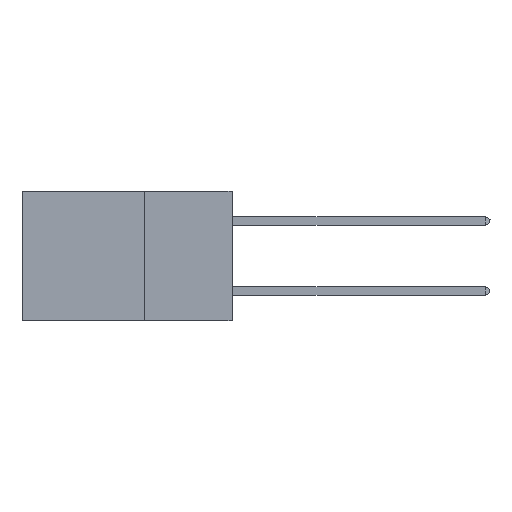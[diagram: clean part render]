
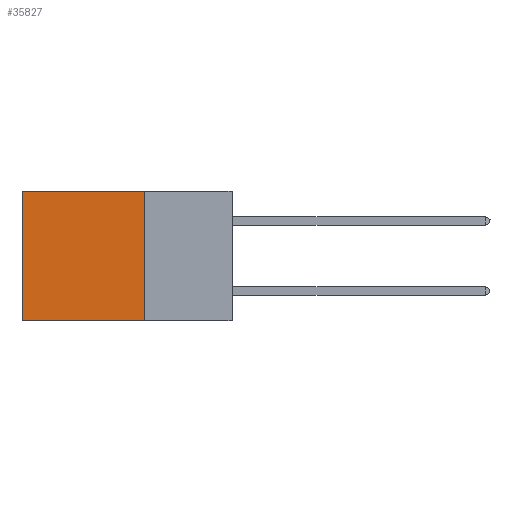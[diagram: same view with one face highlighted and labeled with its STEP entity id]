
A CAD part, left-side view. The second image highlights one B-rep face of the part: STEP entity #35827.
In plain terms, the highlighted planar face has unit normal (-1, 0, 0).
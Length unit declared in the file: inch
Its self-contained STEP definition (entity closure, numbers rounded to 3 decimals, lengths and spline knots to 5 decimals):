
#1956 = LINE ( 'NONE', #14422, #10364 ) ;
#3294 = ORIENTED_EDGE ( 'NONE', *, *, #44660, .T. ) ;
#3341 = DIRECTION ( 'NONE',  ( 0., 1., 0. ) ) ;
#5466 = CARTESIAN_POINT ( 'NONE',  ( 0.2875, 0.6, 0. ) ) ;
#6624 = ORIENTED_EDGE ( 'NONE', *, *, #18819, .F. ) ;
#9872 = EDGE_CURVE ( 'NONE', #36592, #42663, #22064, .T. ) ;
#9989 = VERTEX_POINT ( 'NONE', #5466 ) ;
#10364 = VECTOR ( 'NONE', #18032, 39.37008 ) ;
#11858 = CARTESIAN_POINT ( 'NONE',  ( 0.2875, 0.25, 0. ) ) ;
#13214 = DIRECTION ( 'NONE',  ( 0., 1., 0. ) ) ;
#14422 = CARTESIAN_POINT ( 'NONE',  ( 0.2875, 0.6, 0. ) ) ;
#14888 = DIRECTION ( 'NONE',  ( 0., 0., -1. ) ) ;
#18032 = DIRECTION ( 'NONE',  ( 0., 0., -1. ) ) ;
#18819 = EDGE_CURVE ( 'NONE', #42663, #41972, #26829, .T. ) ;
#19932 = LINE ( 'NONE', #45694, #37537 ) ;
#22064 = LINE ( 'NONE', #11858, #39674 ) ;
#24154 = FACE_OUTER_BOUND ( 'NONE', #41057, .T. ) ;
#26829 = LINE ( 'NONE', #44983, #44404 ) ;
#29022 = PLANE ( 'NONE',  #36742 ) ;
#29556 = DIRECTION ( 'NONE',  ( 0., 0., -1. ) ) ;
#30192 = CARTESIAN_POINT ( 'NONE',  ( 0.2875, 0.25, 0. ) ) ;
#31766 = CARTESIAN_POINT ( 'NONE',  ( 0.2875, 0.25, -0.37 ) ) ;
#35622 = ORIENTED_EDGE ( 'NONE', *, *, #40347, .T. ) ;
#35827 = ADVANCED_FACE ( 'NONE', ( #24154 ), #29022, .F. ) ;
#35907 = CARTESIAN_POINT ( 'NONE',  ( 0.2875, 0.25, 0. ) ) ;
#36064 = DIRECTION ( 'NONE',  ( 1., 0., 0. ) ) ;
#36592 = VERTEX_POINT ( 'NONE', #30192 ) ;
#36742 = AXIS2_PLACEMENT_3D ( 'NONE', #35907, #36064, #14888 ) ;
#37537 = VECTOR ( 'NONE', #3341, 39.37008 ) ;
#37842 = ORIENTED_EDGE ( 'NONE', *, *, #9872, .F. ) ;
#39674 = VECTOR ( 'NONE', #29556, 39.37008 ) ;
#40347 = EDGE_CURVE ( 'NONE', #36592, #9989, #19932, .T. ) ;
#41057 = EDGE_LOOP ( 'NONE', ( #3294, #6624, #37842, #35622 ) ) ;
#41972 = VERTEX_POINT ( 'NONE', #42097 ) ;
#42097 = CARTESIAN_POINT ( 'NONE',  ( 0.2875, 0.6, -0.37 ) ) ;
#42663 = VERTEX_POINT ( 'NONE', #31766 ) ;
#44404 = VECTOR ( 'NONE', #13214, 39.37008 ) ;
#44660 = EDGE_CURVE ( 'NONE', #9989, #41972, #1956, .T. ) ;
#44983 = CARTESIAN_POINT ( 'NONE',  ( 0.2875, 0.25, -0.37 ) ) ;
#45694 = CARTESIAN_POINT ( 'NONE',  ( 0.2875, 0.25, 0. ) ) ;
